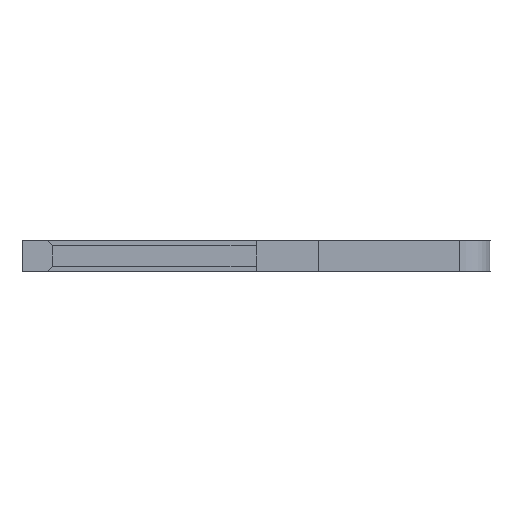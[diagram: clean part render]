
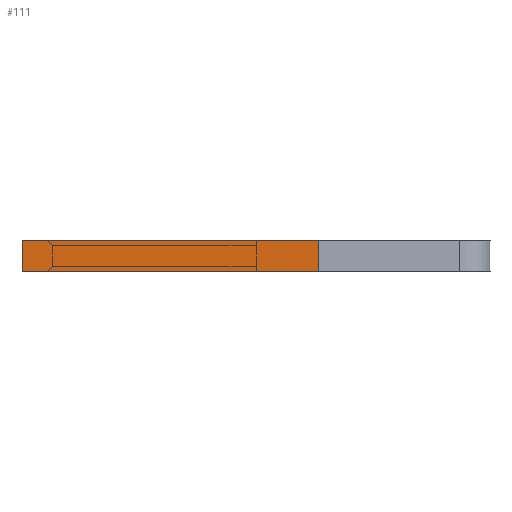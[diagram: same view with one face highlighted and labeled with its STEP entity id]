
A CAD part, left-side view. The second image highlights one B-rep face of the part: STEP entity #111.
In plain terms, the highlighted face is planar.
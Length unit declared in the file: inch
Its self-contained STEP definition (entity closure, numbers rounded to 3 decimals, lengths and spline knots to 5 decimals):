
#111 = ADVANCED_FACE ( 'NONE', ( #2295 ), #382, .F. ) ;
#123 = EDGE_CURVE ( 'NONE', #2268, #2377, #2476, .T. ) ;
#165 = CARTESIAN_POINT ( 'NONE',  ( -0.01, -0.04, -0.04 ) ) ;
#171 = EDGE_CURVE ( 'NONE', #2039, #2377, #387, .T. ) ;
#182 = CARTESIAN_POINT ( 'NONE',  ( 0.01, 0.15, -0.04 ) ) ;
#234 = VERTEX_POINT ( 'NONE', #1014 ) ;
#320 = VECTOR ( 'NONE', #1172, 39.37008 ) ;
#342 = CARTESIAN_POINT ( 'NONE',  ( 0.01, 0.15, -0.04 ) ) ;
#382 = PLANE ( 'NONE',  #909 ) ;
#387 = LINE ( 'NONE', #1169, #1036 ) ;
#479 = EDGE_CURVE ( 'NONE', #234, #2268, #973, .T. ) ;
#543 = LINE ( 'NONE', #2369, #320 ) ;
#575 = VECTOR ( 'NONE', #2165, 39.37008 ) ;
#796 = CARTESIAN_POINT ( 'NONE',  ( -0.01, 0.15, -0.04 ) ) ;
#909 = AXIS2_PLACEMENT_3D ( 'NONE', #1381, #1926, #1758 ) ;
#973 = LINE ( 'NONE', #1985, #2264 ) ;
#1014 = CARTESIAN_POINT ( 'NONE',  ( 0.01, -0.04, -0.04 ) ) ;
#1036 = VECTOR ( 'NONE', #1996, 39.37008 ) ;
#1169 = CARTESIAN_POINT ( 'NONE',  ( -0.01, 0.15, -0.04 ) ) ;
#1172 = DIRECTION ( 'NONE',  ( -1., 0., 0. ) ) ;
#1221 = ORIENTED_EDGE ( 'NONE', *, *, #2463, .T. ) ;
#1381 = CARTESIAN_POINT ( 'NONE',  ( 0.01, 0.15, -0.04 ) ) ;
#1695 = EDGE_LOOP ( 'NONE', ( #1814, #1786, #1940, #1221 ) ) ;
#1758 = DIRECTION ( 'NONE',  ( 1., 0., 0. ) ) ;
#1786 = ORIENTED_EDGE ( 'NONE', *, *, #123, .F. ) ;
#1814 = ORIENTED_EDGE ( 'NONE', *, *, #171, .T. ) ;
#1926 = DIRECTION ( 'NONE',  ( 0., 0., 1. ) ) ;
#1940 = ORIENTED_EDGE ( 'NONE', *, *, #479, .F. ) ;
#1976 = DIRECTION ( 'NONE',  ( 0., 1., 0. ) ) ;
#1985 = CARTESIAN_POINT ( 'NONE',  ( 0.01, 0.15, -0.04 ) ) ;
#1996 = DIRECTION ( 'NONE',  ( 0., 1., 0. ) ) ;
#2039 = VERTEX_POINT ( 'NONE', #165 ) ;
#2165 = DIRECTION ( 'NONE',  ( -1., 0., 0. ) ) ;
#2264 = VECTOR ( 'NONE', #1976, 39.37008 ) ;
#2268 = VERTEX_POINT ( 'NONE', #342 ) ;
#2295 = FACE_OUTER_BOUND ( 'NONE', #1695, .T. ) ;
#2369 = CARTESIAN_POINT ( 'NONE',  ( 0.01, -0.04, -0.04 ) ) ;
#2377 = VERTEX_POINT ( 'NONE', #796 ) ;
#2463 = EDGE_CURVE ( 'NONE', #234, #2039, #543, .T. ) ;
#2476 = LINE ( 'NONE', #182, #575 ) ;
